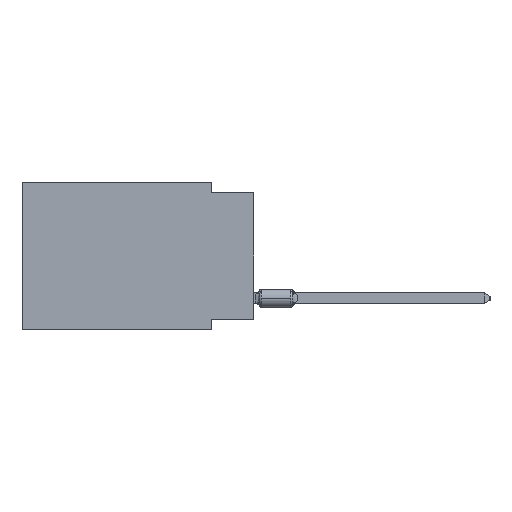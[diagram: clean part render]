
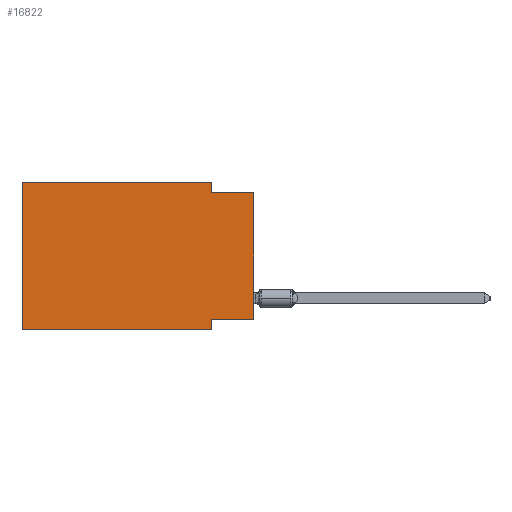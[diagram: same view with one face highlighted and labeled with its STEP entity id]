
A CAD part, left-side view. The second image highlights one B-rep face of the part: STEP entity #16822.
In plain terms, the highlighted planar face has unit normal (-1, 0, 0).
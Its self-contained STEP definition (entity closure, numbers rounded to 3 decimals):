
#668 = CARTESIAN_POINT ( 'NONE',  ( 0., 0., -8.255 ) ) ;
#1049 = CARTESIAN_POINT ( 'NONE',  ( 0., 13.97, 0. ) ) ;
#1470 = CARTESIAN_POINT ( 'NONE',  ( 0., 13.97, 0. ) ) ;
#1654 = LINE ( 'NONE', #21623, #61919 ) ;
#3281 = VERTEX_POINT ( 'NONE', #34087 ) ;
#6568 = DIRECTION ( 'NONE',  ( 0., 1., 0. ) ) ;
#6720 = FACE_OUTER_BOUND ( 'NONE', #36542, .T. ) ;
#6956 = EDGE_CURVE ( 'NONE', #33005, #3281, #17513, .T. ) ;
#7328 = VERTEX_POINT ( 'NONE', #26277 ) ;
#7919 = VECTOR ( 'NONE', #12273, 1000. ) ;
#8753 = CARTESIAN_POINT ( 'NONE',  ( 0., 2.54, 0. ) ) ;
#10561 = DIRECTION ( 'NONE',  ( 0., 0., 1. ) ) ;
#10806 = CARTESIAN_POINT ( 'NONE',  ( 0., 2.54, -0.635 ) ) ;
#11011 = VERTEX_POINT ( 'NONE', #50710 ) ;
#12000 = VECTOR ( 'NONE', #12865, 1000. ) ;
#12273 = DIRECTION ( 'NONE',  ( 0., -1., 0. ) ) ;
#12865 = DIRECTION ( 'NONE',  ( 0., -1., 0. ) ) ;
#12977 = ORIENTED_EDGE ( 'NONE', *, *, #6956, .F. ) ;
#15624 = EDGE_CURVE ( 'NONE', #43694, #11011, #55270, .T. ) ;
#16210 = PLANE ( 'NONE',  #33957 ) ;
#16822 = ADVANCED_FACE ( 'NONE', ( #6720 ), #16210, .F. ) ;
#16932 = CARTESIAN_POINT ( 'NONE',  ( 0., 2.54, -8.255 ) ) ;
#17513 = LINE ( 'NONE', #42422, #7919 ) ;
#18010 = VECTOR ( 'NONE', #63764, 1000. ) ;
#19230 = VECTOR ( 'NONE', #40521, 1000. ) ;
#19785 = ORIENTED_EDGE ( 'NONE', *, *, #43237, .F. ) ;
#20543 = CARTESIAN_POINT ( 'NONE',  ( 0., 2.54, -8.89 ) ) ;
#20831 = ORIENTED_EDGE ( 'NONE', *, *, #57933, .T. ) ;
#21200 = VERTEX_POINT ( 'NONE', #668 ) ;
#21623 = CARTESIAN_POINT ( 'NONE',  ( 0., 0., -8.255 ) ) ;
#23821 = EDGE_CURVE ( 'NONE', #36682, #33005, #35461, .T. ) ;
#24451 = LINE ( 'NONE', #8753, #18010 ) ;
#25482 = EDGE_CURVE ( 'NONE', #21200, #43694, #1654, .T. ) ;
#26277 = CARTESIAN_POINT ( 'NONE',  ( 0., 0., -0.635 ) ) ;
#31216 = VERTEX_POINT ( 'NONE', #10806 ) ;
#33005 = VERTEX_POINT ( 'NONE', #61169 ) ;
#33141 = ORIENTED_EDGE ( 'NONE', *, *, #25482, .F. ) ;
#33957 = AXIS2_PLACEMENT_3D ( 'NONE', #1470, #46015, #41742 ) ;
#34087 = CARTESIAN_POINT ( 'NONE',  ( 0., 2.54, 0. ) ) ;
#35461 = LINE ( 'NONE', #1049, #58655 ) ;
#36542 = EDGE_LOOP ( 'NONE', ( #20831, #50389, #19785, #12977, #37726, #37897, #41382, #33141 ) ) ;
#36682 = VERTEX_POINT ( 'NONE', #51513 ) ;
#37189 = DIRECTION ( 'NONE',  ( 0., 0., 1. ) ) ;
#37726 = ORIENTED_EDGE ( 'NONE', *, *, #23821, .F. ) ;
#37897 = ORIENTED_EDGE ( 'NONE', *, *, #51342, .T. ) ;
#38161 = LINE ( 'NONE', #42434, #48451 ) ;
#40521 = DIRECTION ( 'NONE',  ( 0., 0., -1. ) ) ;
#41382 = ORIENTED_EDGE ( 'NONE', *, *, #15624, .F. ) ;
#41742 = DIRECTION ( 'NONE',  ( 0., 0., -1. ) ) ;
#41923 = LINE ( 'NONE', #45882, #64210 ) ;
#42366 = CARTESIAN_POINT ( 'NONE',  ( 0., 13.97, -8.89 ) ) ;
#42422 = CARTESIAN_POINT ( 'NONE',  ( 0., 13.97, 0. ) ) ;
#42434 = CARTESIAN_POINT ( 'NONE',  ( 0., 0., 0. ) ) ;
#43237 = EDGE_CURVE ( 'NONE', #3281, #31216, #24451, .T. ) ;
#43340 = LINE ( 'NONE', #42366, #12000 ) ;
#43694 = VERTEX_POINT ( 'NONE', #16932 ) ;
#45208 = EDGE_CURVE ( 'NONE', #31216, #7328, #41923, .T. ) ;
#45882 = CARTESIAN_POINT ( 'NONE',  ( 0., 0., -0.635 ) ) ;
#46015 = DIRECTION ( 'NONE',  ( 1., 0., 0. ) ) ;
#48451 = VECTOR ( 'NONE', #37189, 1000. ) ;
#50389 = ORIENTED_EDGE ( 'NONE', *, *, #45208, .F. ) ;
#50710 = CARTESIAN_POINT ( 'NONE',  ( 0., 2.54, -8.89 ) ) ;
#51342 = EDGE_CURVE ( 'NONE', #36682, #11011, #43340, .T. ) ;
#51513 = CARTESIAN_POINT ( 'NONE',  ( 0., 13.97, -8.89 ) ) ;
#55270 = LINE ( 'NONE', #20543, #19230 ) ;
#57933 = EDGE_CURVE ( 'NONE', #21200, #7328, #38161, .T. ) ;
#58655 = VECTOR ( 'NONE', #10561, 1000. ) ;
#61169 = CARTESIAN_POINT ( 'NONE',  ( 0., 13.97, 0. ) ) ;
#61905 = DIRECTION ( 'NONE',  ( 0., -1., 0. ) ) ;
#61919 = VECTOR ( 'NONE', #6568, 1000. ) ;
#63764 = DIRECTION ( 'NONE',  ( 0., 0., -1. ) ) ;
#64210 = VECTOR ( 'NONE', #61905, 1000. ) ;
